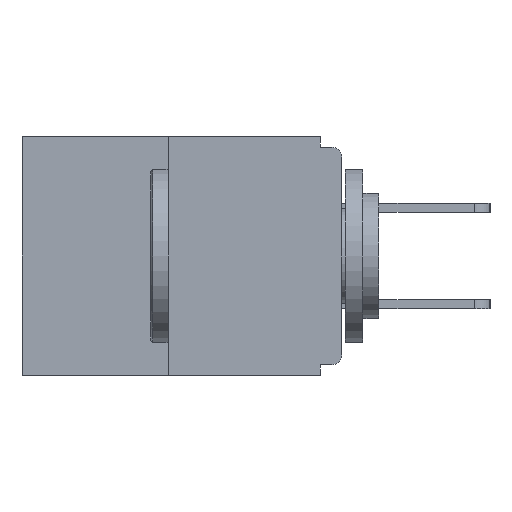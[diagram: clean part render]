
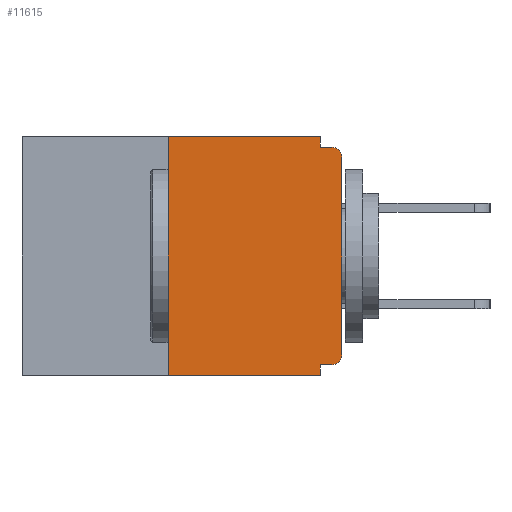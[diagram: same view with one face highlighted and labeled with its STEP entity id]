
A CAD part, left-side view. The second image highlights one B-rep face of the part: STEP entity #11615.
In plain terms, the highlighted planar face has unit normal (-1, 0, 0).
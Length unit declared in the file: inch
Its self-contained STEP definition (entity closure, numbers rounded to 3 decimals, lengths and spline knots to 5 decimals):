
#90 = LINE ( 'NONE', #15255, #24103 ) ;
#165 = AXIS2_PLACEMENT_3D ( 'NONE', #9613, #7694, #23830 ) ;
#776 = CARTESIAN_POINT ( 'NONE',  ( 0., 0.031, 0. ) ) ;
#1492 = CARTESIAN_POINT ( 'NONE',  ( 0., 0., -0.328 ) ) ;
#1657 = VERTEX_POINT ( 'NONE', #9137 ) ;
#2454 = ORIENTED_EDGE ( 'NONE', *, *, #25532, .F. ) ;
#3527 = DIRECTION ( 'NONE',  ( 0., 0., -1. ) ) ;
#3750 = CARTESIAN_POINT ( 'NONE',  ( 0., 0.031, -0.343 ) ) ;
#4420 = VECTOR ( 'NONE', #13868, 39.37008 ) ;
#4614 = ORIENTED_EDGE ( 'NONE', *, *, #30084, .T. ) ;
#4711 = ORIENTED_EDGE ( 'NONE', *, *, #8684, .F. ) ;
#4971 = VECTOR ( 'NONE', #3527, 39.37008 ) ;
#5094 = DIRECTION ( 'NONE',  ( -1., 0., 0. ) ) ;
#5299 = EDGE_CURVE ( 'NONE', #20643, #11294, #11445, .T. ) ;
#5855 = VERTEX_POINT ( 'NONE', #20159 ) ;
#7694 = DIRECTION ( 'NONE',  ( -1., 0., 0. ) ) ;
#7739 = LINE ( 'NONE', #13971, #4420 ) ;
#8684 = EDGE_CURVE ( 'NONE', #19210, #20643, #24940, .T. ) ;
#8786 = CARTESIAN_POINT ( 'NONE',  ( 0., 0.25, 0. ) ) ;
#9137 = CARTESIAN_POINT ( 'NONE',  ( 0., 0.031, -0.328 ) ) ;
#9613 = CARTESIAN_POINT ( 'NONE',  ( 0., 0.015, -0.03 ) ) ;
#10257 = ORIENTED_EDGE ( 'NONE', *, *, #18166, .T. ) ;
#10771 = VERTEX_POINT ( 'NONE', #3750 ) ;
#11138 = LINE ( 'NONE', #26890, #4971 ) ;
#11268 = DIRECTION ( 'NONE',  ( 0., -1., 0. ) ) ;
#11294 = VERTEX_POINT ( 'NONE', #776 ) ;
#11445 = LINE ( 'NONE', #29530, #16570 ) ;
#11463 = VERTEX_POINT ( 'NONE', #22233 ) ;
#11512 = EDGE_CURVE ( 'NONE', #17572, #1657, #11703, .T. ) ;
#11615 = ADVANCED_FACE ( 'NONE', ( #20826 ), #13673, .F. ) ;
#11703 = LINE ( 'NONE', #1492, #26966 ) ;
#12955 = CARTESIAN_POINT ( 'NONE',  ( 0., 0.25, 0. ) ) ;
#13673 = PLANE ( 'NONE',  #23250 ) ;
#13868 = DIRECTION ( 'NONE',  ( 0., -1., 0. ) ) ;
#13971 = CARTESIAN_POINT ( 'NONE',  ( 0., 0., -0.015 ) ) ;
#14576 = CARTESIAN_POINT ( 'NONE',  ( 0., 0.015, -0.015 ) ) ;
#14637 = CARTESIAN_POINT ( 'NONE',  ( 0., 0.015, -0.328 ) ) ;
#15041 = ORIENTED_EDGE ( 'NONE', *, *, #18914, .F. ) ;
#15255 = CARTESIAN_POINT ( 'NONE',  ( 0., 0.46, -0.343 ) ) ;
#15480 = VECTOR ( 'NONE', #27197, 39.37008 ) ;
#16023 = DIRECTION ( 'NONE',  ( 1., 0., 0. ) ) ;
#16570 = VECTOR ( 'NONE', #11268, 39.37008 ) ;
#16761 = CIRCLE ( 'NONE', #25541, 0.015 ) ;
#17389 = CIRCLE ( 'NONE', #165, 0.015 ) ;
#17572 = VERTEX_POINT ( 'NONE', #14637 ) ;
#18036 = DIRECTION ( 'NONE',  ( 0., 0., 1. ) ) ;
#18151 = DIRECTION ( 'NONE',  ( 0., 0., -1. ) ) ;
#18166 = EDGE_CURVE ( 'NONE', #5855, #28786, #17389, .T. ) ;
#18776 = VERTEX_POINT ( 'NONE', #24372 ) ;
#18914 = EDGE_CURVE ( 'NONE', #11294, #11463, #11138, .T. ) ;
#19210 = VERTEX_POINT ( 'NONE', #21231 ) ;
#19323 = CARTESIAN_POINT ( 'NONE',  ( 0., 0.015, -0.313 ) ) ;
#19584 = EDGE_LOOP ( 'NONE', ( #24990, #4711, #4614, #25783, #19590, #28812, #24189, #10257, #2454, #15041 ) ) ;
#19590 = ORIENTED_EDGE ( 'NONE', *, *, #11512, .F. ) ;
#19632 = EDGE_CURVE ( 'NONE', #18776, #5855, #24179, .T. ) ;
#19985 = DIRECTION ( 'NONE',  ( 0., 1., 0. ) ) ;
#20159 = CARTESIAN_POINT ( 'NONE',  ( 0., 0., -0.03 ) ) ;
#20643 = VERTEX_POINT ( 'NONE', #12955 ) ;
#20826 = FACE_OUTER_BOUND ( 'NONE', #19584, .T. ) ;
#21231 = CARTESIAN_POINT ( 'NONE',  ( 0., 0.25, -0.343 ) ) ;
#21252 = EDGE_CURVE ( 'NONE', #17572, #18776, #16761, .T. ) ;
#22019 = VECTOR ( 'NONE', #18036, 39.37008 ) ;
#22070 = DIRECTION ( 'NONE',  ( 0., -1., 0. ) ) ;
#22233 = CARTESIAN_POINT ( 'NONE',  ( 0., 0.031, -0.015 ) ) ;
#23029 = CARTESIAN_POINT ( 'NONE',  ( 0., 0.46, 0. ) ) ;
#23250 = AXIS2_PLACEMENT_3D ( 'NONE', #23029, #16023, #18151 ) ;
#23830 = DIRECTION ( 'NONE',  ( 0., 0., -1. ) ) ;
#23985 = DIRECTION ( 'NONE',  ( 0., 0., -1. ) ) ;
#24103 = VECTOR ( 'NONE', #22070, 39.37008 ) ;
#24179 = LINE ( 'NONE', #24843, #22019 ) ;
#24189 = ORIENTED_EDGE ( 'NONE', *, *, #19632, .T. ) ;
#24201 = VECTOR ( 'NONE', #27444, 39.37008 ) ;
#24372 = CARTESIAN_POINT ( 'NONE',  ( 0., 0., -0.313 ) ) ;
#24782 = CARTESIAN_POINT ( 'NONE',  ( 0., 0.031, -0.343 ) ) ;
#24843 = CARTESIAN_POINT ( 'NONE',  ( 0., 0., 0. ) ) ;
#24940 = LINE ( 'NONE', #8786, #24201 ) ;
#24990 = ORIENTED_EDGE ( 'NONE', *, *, #5299, .F. ) ;
#25532 = EDGE_CURVE ( 'NONE', #11463, #28786, #7739, .T. ) ;
#25541 = AXIS2_PLACEMENT_3D ( 'NONE', #19323, #5094, #23985 ) ;
#25783 = ORIENTED_EDGE ( 'NONE', *, *, #26759, .F. ) ;
#26759 = EDGE_CURVE ( 'NONE', #1657, #10771, #28874, .T. ) ;
#26890 = CARTESIAN_POINT ( 'NONE',  ( 0., 0.031, 0. ) ) ;
#26966 = VECTOR ( 'NONE', #19985, 39.37008 ) ;
#27197 = DIRECTION ( 'NONE',  ( 0., 0., -1. ) ) ;
#27444 = DIRECTION ( 'NONE',  ( 0., 0., 1. ) ) ;
#28786 = VERTEX_POINT ( 'NONE', #14576 ) ;
#28812 = ORIENTED_EDGE ( 'NONE', *, *, #21252, .T. ) ;
#28874 = LINE ( 'NONE', #24782, #15480 ) ;
#29530 = CARTESIAN_POINT ( 'NONE',  ( 0., 0.46, 0. ) ) ;
#30084 = EDGE_CURVE ( 'NONE', #19210, #10771, #90, .T. ) ;
